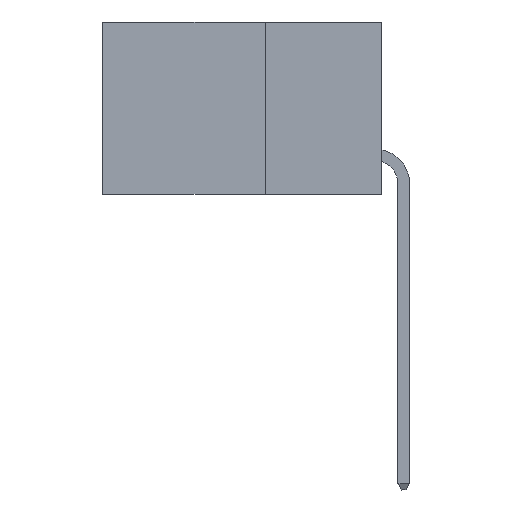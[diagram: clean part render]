
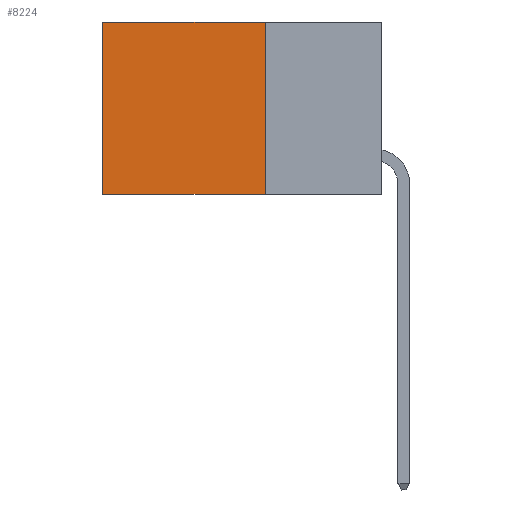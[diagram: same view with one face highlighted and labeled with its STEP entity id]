
A CAD part, left-side view. The second image highlights one B-rep face of the part: STEP entity #8224.
In plain terms, the highlighted planar face has unit normal (-1, 0, 0).
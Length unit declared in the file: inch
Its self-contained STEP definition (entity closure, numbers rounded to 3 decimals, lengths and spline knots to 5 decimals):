
#760 = ORIENTED_EDGE ( 'NONE', *, *, #7352, .T. ) ;
#2903 = VERTEX_POINT ( 'NONE', #4125 ) ;
#3690 = EDGE_CURVE ( 'NONE', #16579, #2903, #5484, .T. ) ;
#4125 = CARTESIAN_POINT ( 'NONE',  ( 0.2875, 0.6, 0. ) ) ;
#4184 = ORIENTED_EDGE ( 'NONE', *, *, #11659, .F. ) ;
#4199 = ORIENTED_EDGE ( 'NONE', *, *, #10018, .F. ) ;
#5484 = LINE ( 'NONE', #15077, #13223 ) ;
#6605 = CARTESIAN_POINT ( 'NONE',  ( 0.2875, 0.25, 0. ) ) ;
#7352 = EDGE_CURVE ( 'NONE', #2903, #11573, #10448, .T. ) ;
#7957 = LINE ( 'NONE', #16247, #19509 ) ;
#8049 = AXIS2_PLACEMENT_3D ( 'NONE', #6605, #8177, #18747 ) ;
#8177 = DIRECTION ( 'NONE',  ( 1., 0., 0. ) ) ;
#8224 = ADVANCED_FACE ( 'NONE', ( #14458 ), #15802, .F. ) ;
#8588 = DIRECTION ( 'NONE',  ( 0., 1., 0. ) ) ;
#9774 = DIRECTION ( 'NONE',  ( 0., 0., -1. ) ) ;
#10018 = EDGE_CURVE ( 'NONE', #17922, #11573, #7957, .T. ) ;
#10448 = LINE ( 'NONE', #10723, #17958 ) ;
#10723 = CARTESIAN_POINT ( 'NONE',  ( 0.2875, 0.6, 0. ) ) ;
#10849 = CARTESIAN_POINT ( 'NONE',  ( 0.2875, 0.25, -0.37 ) ) ;
#11573 = VERTEX_POINT ( 'NONE', #18581 ) ;
#11659 = EDGE_CURVE ( 'NONE', #16579, #17922, #13419, .T. ) ;
#12018 = EDGE_LOOP ( 'NONE', ( #760, #4199, #4184, #12257 ) ) ;
#12257 = ORIENTED_EDGE ( 'NONE', *, *, #3690, .T. ) ;
#12265 = DIRECTION ( 'NONE',  ( 0., 0., -1. ) ) ;
#12968 = VECTOR ( 'NONE', #9774, 39.37008 ) ;
#12981 = CARTESIAN_POINT ( 'NONE',  ( 0.2875, 0.25, 0. ) ) ;
#13223 = VECTOR ( 'NONE', #16572, 39.37008 ) ;
#13419 = LINE ( 'NONE', #14240, #12968 ) ;
#14240 = CARTESIAN_POINT ( 'NONE',  ( 0.2875, 0.25, 0. ) ) ;
#14458 = FACE_OUTER_BOUND ( 'NONE', #12018, .T. ) ;
#15077 = CARTESIAN_POINT ( 'NONE',  ( 0.2875, 0.25, 0. ) ) ;
#15802 = PLANE ( 'NONE',  #8049 ) ;
#16247 = CARTESIAN_POINT ( 'NONE',  ( 0.2875, 0.25, -0.37 ) ) ;
#16572 = DIRECTION ( 'NONE',  ( 0., 1., 0. ) ) ;
#16579 = VERTEX_POINT ( 'NONE', #12981 ) ;
#17922 = VERTEX_POINT ( 'NONE', #10849 ) ;
#17958 = VECTOR ( 'NONE', #12265, 39.37008 ) ;
#18581 = CARTESIAN_POINT ( 'NONE',  ( 0.2875, 0.6, -0.37 ) ) ;
#18747 = DIRECTION ( 'NONE',  ( 0., 0., -1. ) ) ;
#19509 = VECTOR ( 'NONE', #8588, 39.37008 ) ;
